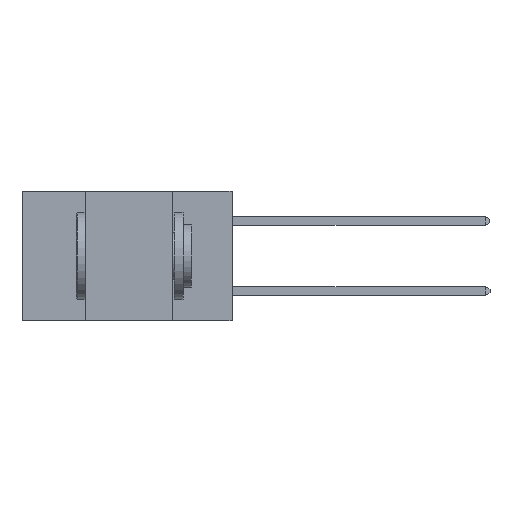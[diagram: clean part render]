
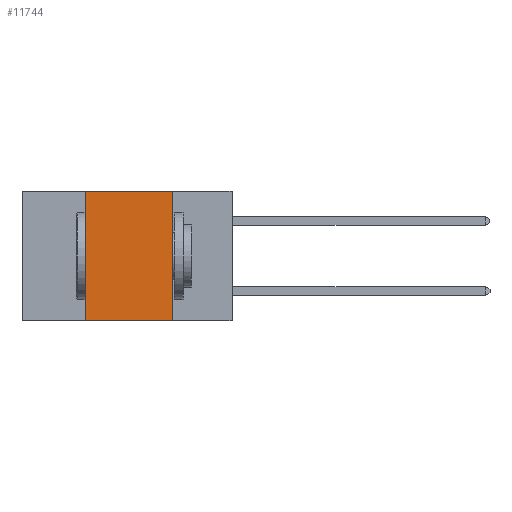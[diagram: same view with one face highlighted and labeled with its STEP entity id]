
A CAD part, left-side view. The second image highlights one B-rep face of the part: STEP entity #11744.
In plain terms, the highlighted planar face has unit normal (-1, 0, 0).
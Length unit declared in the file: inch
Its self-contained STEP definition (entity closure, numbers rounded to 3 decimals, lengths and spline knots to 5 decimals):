
#359 = FACE_OUTER_BOUND ( 'NONE', #20440, .T. ) ;
#1119 = DIRECTION ( 'NONE',  ( 0., -1., 0. ) ) ;
#1339 = VERTEX_POINT ( 'NONE', #10285 ) ;
#1447 = VECTOR ( 'NONE', #1119, 39.37008 ) ;
#1465 = VECTOR ( 'NONE', #8991, 39.37008 ) ;
#1635 = ORIENTED_EDGE ( 'NONE', *, *, #7445, .F. ) ;
#2160 = CARTESIAN_POINT ( 'NONE',  ( 0., 0.17, 0. ) ) ;
#2334 = ORIENTED_EDGE ( 'NONE', *, *, #3750, .F. ) ;
#3494 = VERTEX_POINT ( 'NONE', #2160 ) ;
#3750 = EDGE_CURVE ( 'NONE', #11712, #1339, #14362, .T. ) ;
#3891 = ORIENTED_EDGE ( 'NONE', *, *, #22252, .T. ) ;
#3940 = VECTOR ( 'NONE', #8928, 39.37008 ) ;
#4505 = LINE ( 'NONE', #19575, #3940 ) ;
#5642 = EDGE_CURVE ( 'NONE', #3494, #22683, #19739, .T. ) ;
#6216 = PLANE ( 'NONE',  #20697 ) ;
#7445 = EDGE_CURVE ( 'NONE', #1339, #3494, #4505, .T. ) ;
#8928 = DIRECTION ( 'NONE',  ( 0., -1., 0. ) ) ;
#8991 = DIRECTION ( 'NONE',  ( 0., 0., -1. ) ) ;
#9717 = DIRECTION ( 'NONE',  ( 0., 0., -1. ) ) ;
#10285 = CARTESIAN_POINT ( 'NONE',  ( 0., 0.42, 0. ) ) ;
#11338 = CARTESIAN_POINT ( 'NONE',  ( 0., 0.42, -0.37 ) ) ;
#11443 = LINE ( 'NONE', #22367, #1447 ) ;
#11712 = VERTEX_POINT ( 'NONE', #11338 ) ;
#11744 = ADVANCED_FACE ( 'NONE', ( #359 ), #6216, .F. ) ;
#12216 = ORIENTED_EDGE ( 'NONE', *, *, #5642, .F. ) ;
#13807 = VECTOR ( 'NONE', #16822, 39.37008 ) ;
#14362 = LINE ( 'NONE', #17311, #13807 ) ;
#15007 = CARTESIAN_POINT ( 'NONE',  ( 0., 0.17, -0.37 ) ) ;
#16822 = DIRECTION ( 'NONE',  ( 0., 0., 1. ) ) ;
#17311 = CARTESIAN_POINT ( 'NONE',  ( 0., 0.42, 0. ) ) ;
#18548 = CARTESIAN_POINT ( 'NONE',  ( 0., 0.6, 0. ) ) ;
#19572 = CARTESIAN_POINT ( 'NONE',  ( 0., 0.17, 0. ) ) ;
#19575 = CARTESIAN_POINT ( 'NONE',  ( 0., 0.6, 0. ) ) ;
#19739 = LINE ( 'NONE', #19572, #1465 ) ;
#20298 = DIRECTION ( 'NONE',  ( 1., 0., 0. ) ) ;
#20440 = EDGE_LOOP ( 'NONE', ( #12216, #1635, #2334, #3891 ) ) ;
#20697 = AXIS2_PLACEMENT_3D ( 'NONE', #18548, #20298, #9717 ) ;
#22252 = EDGE_CURVE ( 'NONE', #11712, #22683, #11443, .T. ) ;
#22367 = CARTESIAN_POINT ( 'NONE',  ( 0., 0.6, -0.37 ) ) ;
#22683 = VERTEX_POINT ( 'NONE', #15007 ) ;
